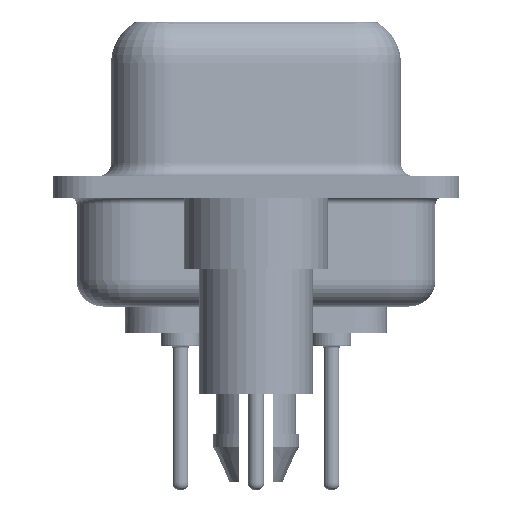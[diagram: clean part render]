
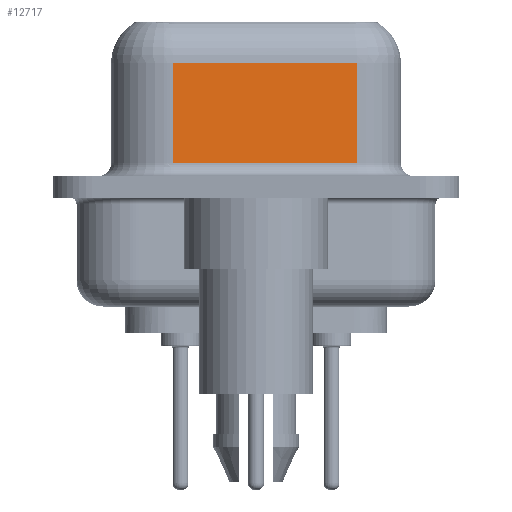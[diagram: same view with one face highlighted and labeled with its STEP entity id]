
A CAD part, left-side view. The second image highlights one B-rep face of the part: STEP entity #12717.
In plain terms, the highlighted planar face has unit normal (-0.985, -0.174, 0).
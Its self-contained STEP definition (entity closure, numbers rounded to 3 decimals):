
#1918 = DIRECTION ( 'NONE',  ( 0.985, 0.174, 0. ) ) ;
#3019 = CARTESIAN_POINT ( 'NONE',  ( 4.43, 3.103, 0.9 ) ) ;
#3341 = CARTESIAN_POINT ( 'NONE',  ( 5.647, -3.797, 4.65 ) ) ;
#4623 = VERTEX_POINT ( 'NONE', #26775 ) ;
#5705 = ORIENTED_EDGE ( 'NONE', *, *, #11022, .T. ) ;
#6007 = EDGE_LOOP ( 'NONE', ( #17296, #5705, #29138, #25678 ) ) ;
#6126 = CARTESIAN_POINT ( 'NONE',  ( 4.43, 3.103, 4.65 ) ) ;
#6723 = CARTESIAN_POINT ( 'NONE',  ( 4.43, 3.103, 6.4 ) ) ;
#7208 = EDGE_CURVE ( 'NONE', #7478, #4623, #14943, .T. ) ;
#7478 = VERTEX_POINT ( 'NONE', #18865 ) ;
#8345 = VERTEX_POINT ( 'NONE', #3019 ) ;
#9781 = DIRECTION ( 'NONE',  ( 0., 0., -1. ) ) ;
#11022 = EDGE_CURVE ( 'NONE', #7478, #11324, #15742, .T. ) ;
#11324 = VERTEX_POINT ( 'NONE', #6126 ) ;
#11835 = EDGE_CURVE ( 'NONE', #8345, #4623, #25810, .T. ) ;
#12717 = ADVANCED_FACE ( 'NONE', ( #19555 ), #15033, .F. ) ;
#14943 = LINE ( 'NONE', #25398, #24394 ) ;
#15033 = PLANE ( 'NONE',  #22005 ) ;
#15742 = LINE ( 'NONE', #3341, #20247 ) ;
#17296 = ORIENTED_EDGE ( 'NONE', *, *, #7208, .F. ) ;
#18865 = CARTESIAN_POINT ( 'NONE',  ( 5.647, -3.797, 4.65 ) ) ;
#19555 = FACE_OUTER_BOUND ( 'NONE', #6007, .T. ) ;
#19799 = LINE ( 'NONE', #6723, #32784 ) ;
#20247 = VECTOR ( 'NONE', #32378, 1000. ) ;
#22005 = AXIS2_PLACEMENT_3D ( 'NONE', #25487, #1918, #22933 ) ;
#22933 = DIRECTION ( 'NONE',  ( -0.174, 0.985, 0. ) ) ;
#24394 = VECTOR ( 'NONE', #9781, 1000. ) ;
#25398 = CARTESIAN_POINT ( 'NONE',  ( 5.647, -3.797, 6.4 ) ) ;
#25487 = CARTESIAN_POINT ( 'NONE',  ( 5.647, -3.797, 6.4 ) ) ;
#25678 = ORIENTED_EDGE ( 'NONE', *, *, #11835, .T. ) ;
#25810 = LINE ( 'NONE', #26137, #31247 ) ;
#26137 = CARTESIAN_POINT ( 'NONE',  ( 5.647, -3.797, 0.9 ) ) ;
#26161 = EDGE_CURVE ( 'NONE', #11324, #8345, #19799, .T. ) ;
#26775 = CARTESIAN_POINT ( 'NONE',  ( 5.647, -3.797, 0.9 ) ) ;
#27681 = DIRECTION ( 'NONE',  ( 0., 0., -1. ) ) ;
#29138 = ORIENTED_EDGE ( 'NONE', *, *, #26161, .T. ) ;
#31247 = VECTOR ( 'NONE', #33829, 1000. ) ;
#32378 = DIRECTION ( 'NONE',  ( -0.174, 0.985, 0. ) ) ;
#32784 = VECTOR ( 'NONE', #27681, 1000. ) ;
#33829 = DIRECTION ( 'NONE',  ( 0.174, -0.985, 0. ) ) ;
